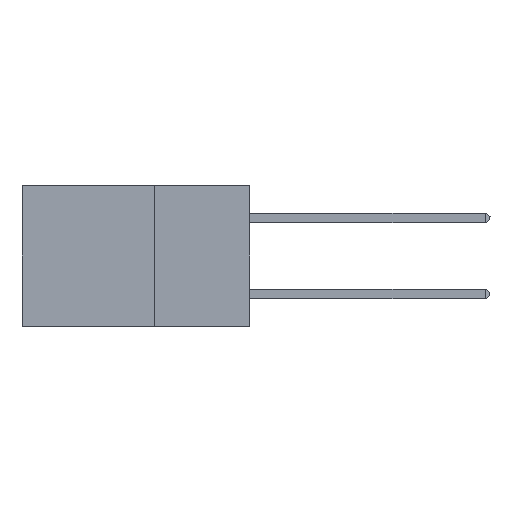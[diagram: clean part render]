
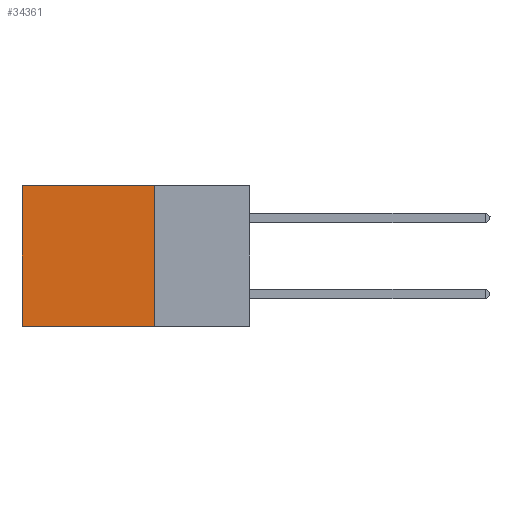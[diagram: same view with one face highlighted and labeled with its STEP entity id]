
A CAD part, left-side view. The second image highlights one B-rep face of the part: STEP entity #34361.
In plain terms, the highlighted planar face has unit normal (-1, 0, 0).
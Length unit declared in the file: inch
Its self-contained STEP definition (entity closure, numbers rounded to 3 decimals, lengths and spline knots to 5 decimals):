
#288 = DIRECTION ( 'NONE',  ( 1., 0., 0. ) ) ;
#2052 = VECTOR ( 'NONE', #35725, 39.37008 ) ;
#2196 = FACE_OUTER_BOUND ( 'NONE', #36159, .T. ) ;
#3347 = CARTESIAN_POINT ( 'NONE',  ( 0.2875, 0.6, 0. ) ) ;
#3901 = CARTESIAN_POINT ( 'NONE',  ( 0.2875, 0.6, 0. ) ) ;
#4625 = LINE ( 'NONE', #40692, #33769 ) ;
#5157 = VERTEX_POINT ( 'NONE', #11022 ) ;
#9886 = VECTOR ( 'NONE', #29190, 39.37008 ) ;
#11022 = CARTESIAN_POINT ( 'NONE',  ( 0.2875, 0.6, -0.37 ) ) ;
#12263 = CARTESIAN_POINT ( 'NONE',  ( 0.2875, 0.25, 0. ) ) ;
#14926 = CARTESIAN_POINT ( 'NONE',  ( 0.2875, 0.25, -0.37 ) ) ;
#15599 = AXIS2_PLACEMENT_3D ( 'NONE', #18583, #288, #25935 ) ;
#18583 = CARTESIAN_POINT ( 'NONE',  ( 0.2875, 0.25, 0. ) ) ;
#18916 = DIRECTION ( 'NONE',  ( 0., 1., 0. ) ) ;
#20332 = EDGE_CURVE ( 'NONE', #30694, #5157, #25485, .T. ) ;
#21540 = ORIENTED_EDGE ( 'NONE', *, *, #42379, .F. ) ;
#21834 = CARTESIAN_POINT ( 'NONE',  ( 0.2875, 0.25, 0. ) ) ;
#22736 = LINE ( 'NONE', #43002, #2052 ) ;
#25301 = DIRECTION ( 'NONE',  ( 0., 0., -1. ) ) ;
#25485 = LINE ( 'NONE', #3347, #44760 ) ;
#25935 = DIRECTION ( 'NONE',  ( 0., 0., -1. ) ) ;
#26196 = ORIENTED_EDGE ( 'NONE', *, *, #20332, .T. ) ;
#26576 = ORIENTED_EDGE ( 'NONE', *, *, #40051, .T. ) ;
#29190 = DIRECTION ( 'NONE',  ( 0., 0., -1. ) ) ;
#29320 = LINE ( 'NONE', #21834, #9886 ) ;
#30694 = VERTEX_POINT ( 'NONE', #3901 ) ;
#33769 = VECTOR ( 'NONE', #18916, 39.37008 ) ;
#34361 = ADVANCED_FACE ( 'NONE', ( #2196 ), #40387, .F. ) ;
#35725 = DIRECTION ( 'NONE',  ( 0., 1., 0. ) ) ;
#36159 = EDGE_LOOP ( 'NONE', ( #26196, #21540, #46842, #26576 ) ) ;
#36865 = VERTEX_POINT ( 'NONE', #14926 ) ;
#40051 = EDGE_CURVE ( 'NONE', #43305, #30694, #4625, .T. ) ;
#40387 = PLANE ( 'NONE',  #15599 ) ;
#40692 = CARTESIAN_POINT ( 'NONE',  ( 0.2875, 0.25, 0. ) ) ;
#42379 = EDGE_CURVE ( 'NONE', #36865, #5157, #22736, .T. ) ;
#43002 = CARTESIAN_POINT ( 'NONE',  ( 0.2875, 0.25, -0.37 ) ) ;
#43305 = VERTEX_POINT ( 'NONE', #12263 ) ;
#44760 = VECTOR ( 'NONE', #25301, 39.37008 ) ;
#45470 = EDGE_CURVE ( 'NONE', #43305, #36865, #29320, .T. ) ;
#46842 = ORIENTED_EDGE ( 'NONE', *, *, #45470, .F. ) ;
